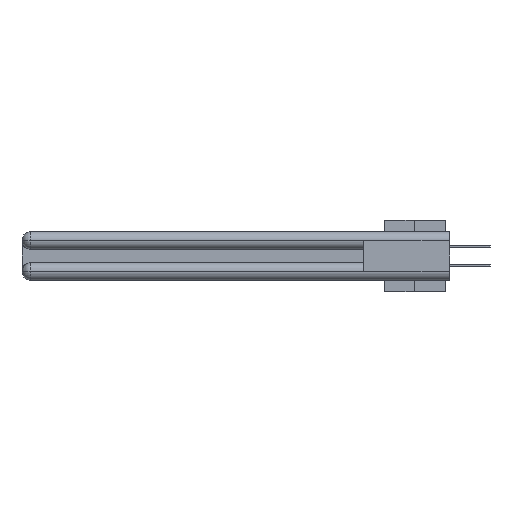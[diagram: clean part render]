
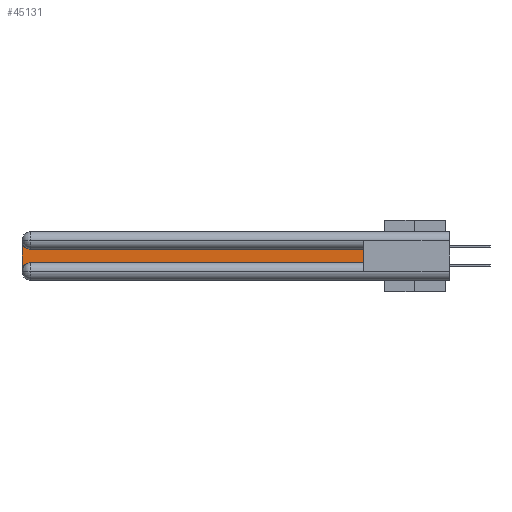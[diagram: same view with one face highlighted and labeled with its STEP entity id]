
A CAD part, left-side view. The second image highlights one B-rep face of the part: STEP entity #45131.
In plain terms, the highlighted planar face has unit normal (-1, 0, 0).
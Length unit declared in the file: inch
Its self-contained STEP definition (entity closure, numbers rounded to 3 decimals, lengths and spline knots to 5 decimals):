
#2165 = LINE ( 'NONE', #33204, #39728 ) ;
#3264 = CARTESIAN_POINT ( 'NONE',  ( 0.075, 3., -0.2775 ) ) ;
#3998 = CARTESIAN_POINT ( 'NONE',  ( 0.075, 2.94, -0.2775 ) ) ;
#5852 = CARTESIAN_POINT ( 'NONE',  ( 0.075, 2.94, -0.1225 ) ) ;
#6520 = VECTOR ( 'NONE', #30100, 39.37008 ) ;
#7552 = CARTESIAN_POINT ( 'NONE',  ( 0.075, 2.94, -0.2175 ) ) ;
#7948 = VERTEX_POINT ( 'NONE', #32261 ) ;
#9232 = VERTEX_POINT ( 'NONE', #7552 ) ;
#9655 = ORIENTED_EDGE ( 'NONE', *, *, #28316, .T. ) ;
#10512 = CARTESIAN_POINT ( 'NONE',  ( 0.075, 0.6, -0.2175 ) ) ;
#11026 = DIRECTION ( 'NONE',  ( 1., 0., 0. ) ) ;
#13480 = AXIS2_PLACEMENT_3D ( 'NONE', #45260, #45559, #23441 ) ;
#13723 = DIRECTION ( 'NONE',  ( 0., 0., -1. ) ) ;
#14358 = DIRECTION ( 'NONE',  ( 0., 0., -1. ) ) ;
#14428 = AXIS2_PLACEMENT_3D ( 'NONE', #3998, #11026, #29797 ) ;
#14799 = VERTEX_POINT ( 'NONE', #42423 ) ;
#15526 = EDGE_CURVE ( 'NONE', #17706, #7948, #21840, .T. ) ;
#17662 = PLANE ( 'NONE',  #44846 ) ;
#17706 = VERTEX_POINT ( 'NONE', #44992 ) ;
#17990 = FACE_OUTER_BOUND ( 'NONE', #33056, .T. ) ;
#18330 = CIRCLE ( 'NONE', #14428, 0.06 ) ;
#21840 = LINE ( 'NONE', #10512, #46340 ) ;
#23441 = DIRECTION ( 'NONE',  ( 0., 0., -1. ) ) ;
#27491 = VERTEX_POINT ( 'NONE', #3264 ) ;
#28044 = DIRECTION ( 'NONE',  ( 0., 0., 1. ) ) ;
#28316 = EDGE_CURVE ( 'NONE', #27491, #9232, #18330, .T. ) ;
#29518 = ORIENTED_EDGE ( 'NONE', *, *, #15526, .T. ) ;
#29725 = DIRECTION ( 'NONE',  ( 0., 1., 0. ) ) ;
#29797 = DIRECTION ( 'NONE',  ( 0., 0., -1. ) ) ;
#30100 = DIRECTION ( 'NONE',  ( 0., -1., 0. ) ) ;
#30567 = CARTESIAN_POINT ( 'NONE',  ( 0.075, 0.6, -0.2175 ) ) ;
#31048 = LINE ( 'NONE', #30567, #6520 ) ;
#31109 = LINE ( 'NONE', #46343, #37349 ) ;
#32261 = CARTESIAN_POINT ( 'NONE',  ( 0.075, 0.6, -0.1225 ) ) ;
#32556 = EDGE_CURVE ( 'NONE', #14799, #27491, #31109, .T. ) ;
#32713 = ORIENTED_EDGE ( 'NONE', *, *, #36809, .T. ) ;
#32807 = VERTEX_POINT ( 'NONE', #5852 ) ;
#33056 = EDGE_LOOP ( 'NONE', ( #41354, #33862, #36307, #9655, #32713, #29518 ) ) ;
#33204 = CARTESIAN_POINT ( 'NONE',  ( 0.075, 0.6, -0.1225 ) ) ;
#33862 = ORIENTED_EDGE ( 'NONE', *, *, #35692, .T. ) ;
#34795 = DIRECTION ( 'NONE',  ( 1., 0., 0. ) ) ;
#35339 = EDGE_CURVE ( 'NONE', #7948, #32807, #2165, .T. ) ;
#35692 = EDGE_CURVE ( 'NONE', #32807, #14799, #37419, .T. ) ;
#36213 = CARTESIAN_POINT ( 'NONE',  ( 0.075, 3., -0.1225 ) ) ;
#36307 = ORIENTED_EDGE ( 'NONE', *, *, #32556, .T. ) ;
#36809 = EDGE_CURVE ( 'NONE', #9232, #17706, #31048, .T. ) ;
#37349 = VECTOR ( 'NONE', #13723, 39.37008 ) ;
#37419 = CIRCLE ( 'NONE', #13480, 0.06 ) ;
#39728 = VECTOR ( 'NONE', #29725, 39.37008 ) ;
#41354 = ORIENTED_EDGE ( 'NONE', *, *, #35339, .T. ) ;
#42423 = CARTESIAN_POINT ( 'NONE',  ( 0.075, 3., -0.0625 ) ) ;
#44846 = AXIS2_PLACEMENT_3D ( 'NONE', #36213, #34795, #14358 ) ;
#44992 = CARTESIAN_POINT ( 'NONE',  ( 0.075, 0.6, -0.2175 ) ) ;
#45131 = ADVANCED_FACE ( 'NONE', ( #17990 ), #17662, .F. ) ;
#45260 = CARTESIAN_POINT ( 'NONE',  ( 0.075, 2.94, -0.0625 ) ) ;
#45559 = DIRECTION ( 'NONE',  ( 1., 0., 0. ) ) ;
#46340 = VECTOR ( 'NONE', #28044, 39.37008 ) ;
#46343 = CARTESIAN_POINT ( 'NONE',  ( 0.075, 3., -0.2175 ) ) ;
